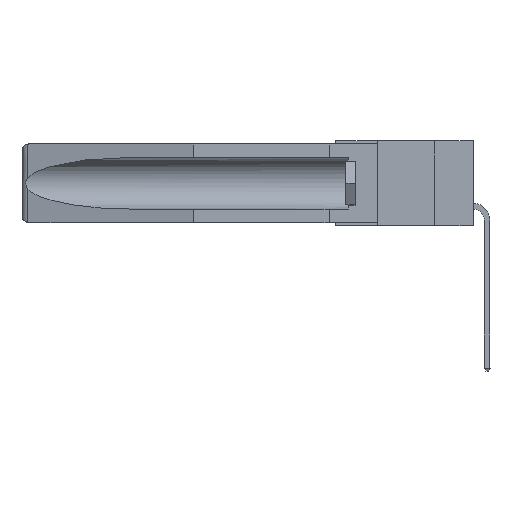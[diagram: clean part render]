
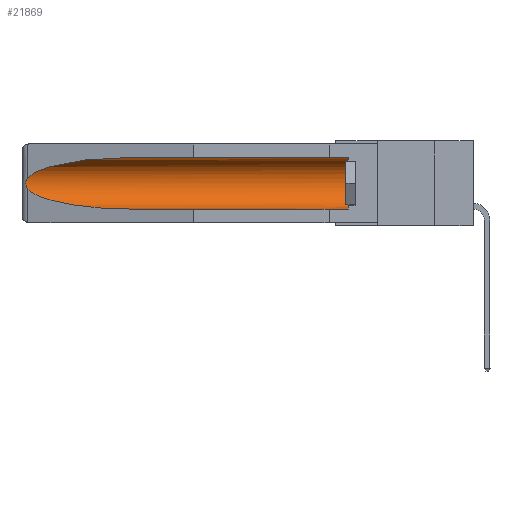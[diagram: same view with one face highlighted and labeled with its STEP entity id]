
A CAD part, left-side view. The second image highlights one B-rep face of the part: STEP entity #21869.
In plain terms, the highlighted cylindrical face has radius 2.857 mm (diameter 5.715 mm), a partial arc.
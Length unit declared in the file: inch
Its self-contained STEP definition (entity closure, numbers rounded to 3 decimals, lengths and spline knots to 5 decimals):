
#340 = DIRECTION ( 'NONE',  ( 0., 1., 0. ) ) ;
#865 = ORIENTED_EDGE ( 'NONE', *, *, #20671, .T. ) ;
#984 = VERTEX_POINT ( 'NONE', #8716 ) ;
#2083 = VERTEX_POINT ( 'NONE', #27998 ) ;
#2193 = CARTESIAN_POINT ( 'NONE',  ( 0.2675, 1.53308, -0.17534 ) ) ;
#2289 = CARTESIAN_POINT ( 'NONE',  ( 0.26654, 1.53092, -0.15636 ) ) ;
#4465 = LINE ( 'NONE', #12252, #6177 ) ;
#4673 = AXIS2_PLACEMENT_3D ( 'NONE', #26540, #9017, #24535 ) ;
#5003 = CARTESIAN_POINT ( 'NONE',  ( 0.155, 1.07973, -0.059 ) ) ;
#5261 = VERTEX_POINT ( 'NONE', #10305 ) ;
#5509 = CARTESIAN_POINT ( 'NONE',  ( 0.26537, 1.52718, -0.14972 ) ) ;
#6177 = VECTOR ( 'NONE', #16930, 39.37008 ) ;
#6804 = CARTESIAN_POINT ( 'NONE',  ( 0.2675, 1.53308, -0.16763 ) ) ;
#6941 = EDGE_CURVE ( 'NONE', #5261, #2083, #27726, .T. ) ;
#7781 = EDGE_CURVE ( 'NONE', #12495, #14460, #8673, .T. ) ;
#7961 = ORIENTED_EDGE ( 'NONE', *, *, #28223, .T. ) ;
#8673 = LINE ( 'NONE', #18284, #22384 ) ;
#8716 = CARTESIAN_POINT ( 'NONE',  ( 0.155, 0.126, -0.284 ) ) ;
#9017 = DIRECTION ( 'NONE',  ( 0., -1., 0. ) ) ;
#9044 = CARTESIAN_POINT ( 'NONE',  ( 0.155, -0.30754, -0.1715 ) ) ;
#9337 = CARTESIAN_POINT ( 'NONE',  ( 0.25451, 1.48313, -0.09465 ) ) ;
#10305 = CARTESIAN_POINT ( 'NONE',  ( 0.26537, 1.52718, -0.14972 ) ) ;
#11412 = FACE_OUTER_BOUND ( 'NONE', #26676, .T. ) ;
#11705 = AXIS2_PLACEMENT_3D ( 'NONE', #9044, #340, #17875 ) ;
#12088 = CARTESIAN_POINT ( 'NONE',  ( 0.25451, 1.48313, -0.24835 ) ) ;
#12252 = CARTESIAN_POINT ( 'NONE',  ( 0.155, -0.30754, -0.284 ) ) ;
#12495 = VERTEX_POINT ( 'NONE', #26006 ) ;
#13041 = CARTESIAN_POINT ( 'NONE',  ( 0.26537, 1.52718, -0.19328 ) ) ;
#13321 = CARTESIAN_POINT ( 'NONE',  ( 0.26597, 1.52961, -0.15275 ) ) ;
#13337 =( BOUNDED_CURVE ( )  B_SPLINE_CURVE ( 3, ( #27575, #12088, #14185, #16382 ),
 .UNSPECIFIED., .F., .F. ) 
 B_SPLINE_CURVE_WITH_KNOTS ( ( 4, 4 ),
 ( 0.1948, 1.5708 ),
 .UNSPECIFIED. ) 
 CURVE ( )  GEOMETRIC_REPRESENTATION_ITEM ( )  RATIONAL_B_SPLINE_CURVE ( ( 1., 0.848, 0.848, 1. ) ) 
 REPRESENTATION_ITEM ( '' )  );
#14185 = CARTESIAN_POINT ( 'NONE',  ( 0.21114, 1.30732, -0.284 ) ) ;
#14393 = VERTEX_POINT ( 'NONE', #19974 ) ;
#14460 = VERTEX_POINT ( 'NONE', #26659 ) ;
#15325 = EDGE_CURVE ( 'NONE', #2083, #14393, #13337, .T. ) ;
#15327 = CARTESIAN_POINT ( 'NONE',  ( 0.2673, 1.5327, -0.16383 ) ) ;
#15797 =( BOUNDED_CURVE ( )  B_SPLINE_CURVE ( 3, ( #5003, #20333, #9337, #5509 ),
 .UNSPECIFIED., .F., .F. ) 
 B_SPLINE_CURVE_WITH_KNOTS ( ( 4, 4 ),
 ( 4.71239, 6.08839 ),
 .UNSPECIFIED. ) 
 CURVE ( )  GEOMETRIC_REPRESENTATION_ITEM ( )  RATIONAL_B_SPLINE_CURVE ( ( 1., 0.848, 0.848, 1. ) ) 
 REPRESENTATION_ITEM ( '' )  );
#16382 = CARTESIAN_POINT ( 'NONE',  ( 0.155, 1.07973, -0.284 ) ) ;
#16930 = DIRECTION ( 'NONE',  ( 0., 1., 0. ) ) ;
#17875 = DIRECTION ( 'NONE',  ( 0., 0., 1. ) ) ;
#18192 = DIRECTION ( 'NONE',  ( 0., 1., 0. ) ) ;
#18284 = CARTESIAN_POINT ( 'NONE',  ( 0.155, -0.30754, -0.059 ) ) ;
#19833 = CARTESIAN_POINT ( 'NONE',  ( 0.2673, 1.53269, -0.17917 ) ) ;
#19974 = CARTESIAN_POINT ( 'NONE',  ( 0.155, 1.07973, -0.284 ) ) ;
#20007 = CIRCLE ( 'NONE', #4673, 0.1125 ) ;
#20333 = CARTESIAN_POINT ( 'NONE',  ( 0.21114, 1.30732, -0.059 ) ) ;
#20671 = EDGE_CURVE ( 'NONE', #984, #12495, #20007, .T. ) ;
#20731 = ORIENTED_EDGE ( 'NONE', *, *, #15325, .T. ) ;
#21869 = ADVANCED_FACE ( 'NONE', ( #11412 ), #25097, .F. ) ;
#22384 = VECTOR ( 'NONE', #18192, 39.37008 ) ;
#23242 = ORIENTED_EDGE ( 'NONE', *, *, #6941, .T. ) ;
#23399 = ORIENTED_EDGE ( 'NONE', *, *, #7781, .T. ) ;
#24315 = CARTESIAN_POINT ( 'NONE',  ( 0.26597, 1.5296, -0.19026 ) ) ;
#24535 = DIRECTION ( 'NONE',  ( 0., 0., 1. ) ) ;
#25097 = CYLINDRICAL_SURFACE ( 'NONE', #11705, 0.1125 ) ;
#25311 = ORIENTED_EDGE ( 'NONE', *, *, #27115, .F. ) ;
#26006 = CARTESIAN_POINT ( 'NONE',  ( 0.155, 0.126, -0.059 ) ) ;
#26129 = CARTESIAN_POINT ( 'NONE',  ( 0.26537, 1.52718, -0.14972 ) ) ;
#26419 = CARTESIAN_POINT ( 'NONE',  ( 0.26655, 1.53094, -0.18657 ) ) ;
#26540 = CARTESIAN_POINT ( 'NONE',  ( 0.155, 0.126, -0.1715 ) ) ;
#26659 = CARTESIAN_POINT ( 'NONE',  ( 0.155, 1.07973, -0.059 ) ) ;
#26676 = EDGE_LOOP ( 'NONE', ( #7961, #23242, #20731, #25311, #865, #23399 ) ) ;
#27115 = EDGE_CURVE ( 'NONE', #984, #14393, #4465, .T. ) ;
#27575 = CARTESIAN_POINT ( 'NONE',  ( 0.26537, 1.52718, -0.19328 ) ) ;
#27726 = B_SPLINE_CURVE_WITH_KNOTS ( 'NONE', 3,
 ( #26129, #13321, #2289, #15327, #6804, #2193, #19833, #26419, #24315, #13041 ),
 .UNSPECIFIED., .F., .F.,
 ( 4, 2, 2, 2, 4 ),
 ( 0., 0.00029, 0.00058, 0.00087, 0.00117 ),
 .UNSPECIFIED. ) ;
#27998 = CARTESIAN_POINT ( 'NONE',  ( 0.26537, 1.52718, -0.19328 ) ) ;
#28223 = EDGE_CURVE ( 'NONE', #14460, #5261, #15797, .T. ) ;
